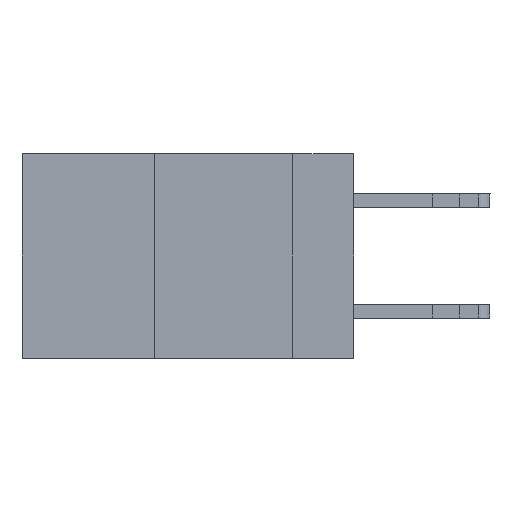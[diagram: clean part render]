
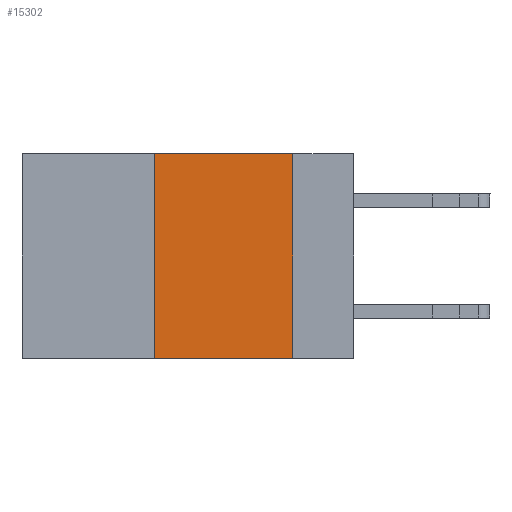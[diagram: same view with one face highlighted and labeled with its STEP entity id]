
A CAD part, left-side view. The second image highlights one B-rep face of the part: STEP entity #15302.
In plain terms, the highlighted planar face has unit normal (-1, 0, 0).
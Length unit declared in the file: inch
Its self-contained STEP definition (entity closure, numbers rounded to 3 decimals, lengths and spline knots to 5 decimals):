
#818 = DIRECTION ( 'NONE',  ( 0., -1., 0. ) ) ;
#1764 = VERTEX_POINT ( 'NONE', #15615 ) ;
#2701 = DIRECTION ( 'NONE',  ( 0., 0., 1. ) ) ;
#2735 = CARTESIAN_POINT ( 'NONE',  ( 0., 0.6, -0.37 ) ) ;
#3657 = VERTEX_POINT ( 'NONE', #20453 ) ;
#4643 = LINE ( 'NONE', #2735, #9126 ) ;
#4899 = DIRECTION ( 'NONE',  ( 0., 0., -1. ) ) ;
#5646 = VERTEX_POINT ( 'NONE', #7938 ) ;
#6636 = LINE ( 'NONE', #8531, #23262 ) ;
#7305 = PLANE ( 'NONE',  #7918 ) ;
#7727 = LINE ( 'NONE', #21349, #24548 ) ;
#7918 = AXIS2_PLACEMENT_3D ( 'NONE', #14953, #24233, #4899 ) ;
#7938 = CARTESIAN_POINT ( 'NONE',  ( 0., 0.11, -0.37 ) ) ;
#8531 = CARTESIAN_POINT ( 'NONE',  ( 0., 0.36, 0. ) ) ;
#8703 = FACE_OUTER_BOUND ( 'NONE', #12031, .T. ) ;
#9126 = VECTOR ( 'NONE', #818, 39.37008 ) ;
#9426 = ORIENTED_EDGE ( 'NONE', *, *, #21074, .F. ) ;
#9643 = DIRECTION ( 'NONE',  ( 0., 0., -1. ) ) ;
#10360 = EDGE_CURVE ( 'NONE', #1764, #3657, #17266, .T. ) ;
#12031 = EDGE_LOOP ( 'NONE', ( #15565, #16485, #9426, #14277 ) ) ;
#12917 = EDGE_CURVE ( 'NONE', #3657, #5646, #7727, .T. ) ;
#13323 = CARTESIAN_POINT ( 'NONE',  ( 0., 0.6, 0. ) ) ;
#13454 = EDGE_CURVE ( 'NONE', #22837, #5646, #4643, .T. ) ;
#14277 = ORIENTED_EDGE ( 'NONE', *, *, #13454, .T. ) ;
#14953 = CARTESIAN_POINT ( 'NONE',  ( 0., 0.6, 0. ) ) ;
#15302 = ADVANCED_FACE ( 'NONE', ( #8703 ), #7305, .F. ) ;
#15565 = ORIENTED_EDGE ( 'NONE', *, *, #12917, .F. ) ;
#15615 = CARTESIAN_POINT ( 'NONE',  ( 0., 0.36, 0. ) ) ;
#16485 = ORIENTED_EDGE ( 'NONE', *, *, #10360, .F. ) ;
#17266 = LINE ( 'NONE', #13323, #18350 ) ;
#18350 = VECTOR ( 'NONE', #20828, 39.37008 ) ;
#20453 = CARTESIAN_POINT ( 'NONE',  ( 0., 0.11, 0. ) ) ;
#20828 = DIRECTION ( 'NONE',  ( 0., -1., 0. ) ) ;
#20981 = CARTESIAN_POINT ( 'NONE',  ( 0., 0.36, -0.37 ) ) ;
#21074 = EDGE_CURVE ( 'NONE', #22837, #1764, #6636, .T. ) ;
#21349 = CARTESIAN_POINT ( 'NONE',  ( 0., 0.11, 0. ) ) ;
#22837 = VERTEX_POINT ( 'NONE', #20981 ) ;
#23262 = VECTOR ( 'NONE', #2701, 39.37008 ) ;
#24233 = DIRECTION ( 'NONE',  ( 1., 0., 0. ) ) ;
#24548 = VECTOR ( 'NONE', #9643, 39.37008 ) ;
